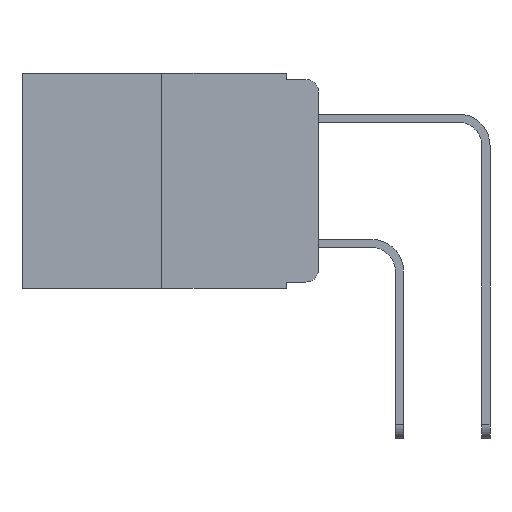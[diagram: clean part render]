
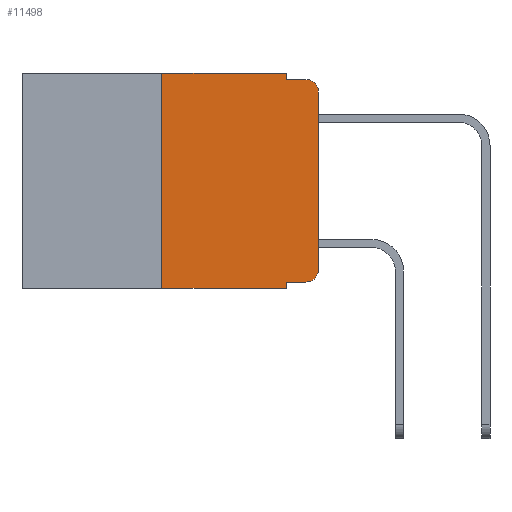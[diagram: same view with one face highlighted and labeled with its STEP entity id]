
A CAD part, left-side view. The second image highlights one B-rep face of the part: STEP entity #11498.
In plain terms, the highlighted planar face has unit normal (-1, 0, 0).
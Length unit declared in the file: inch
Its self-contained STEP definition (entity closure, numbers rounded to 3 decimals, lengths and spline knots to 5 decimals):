
#82 = CARTESIAN_POINT ( 'NONE',  ( 0., 0.051, -0.01 ) ) ;
#469 = CARTESIAN_POINT ( 'NONE',  ( 0., 0.051, -0.333 ) ) ;
#760 = CIRCLE ( 'NONE', #11739, 0.02 ) ;
#832 = PLANE ( 'NONE',  #13525 ) ;
#1111 = EDGE_CURVE ( 'NONE', #13095, #7187, #3518, .T. ) ;
#1128 = ORIENTED_EDGE ( 'NONE', *, *, #9737, .F. ) ;
#1311 = VECTOR ( 'NONE', #10283, 39.37008 ) ;
#1723 = FACE_OUTER_BOUND ( 'NONE', #11784, .T. ) ;
#1800 = EDGE_CURVE ( 'NONE', #10141, #4772, #9819, .T. ) ;
#1827 = CARTESIAN_POINT ( 'NONE',  ( 0., 0.25, 0. ) ) ;
#1835 = VERTEX_POINT ( 'NONE', #9747 ) ;
#1875 = DIRECTION ( 'NONE',  ( 1., 0., 0. ) ) ;
#1890 = DIRECTION ( 'NONE',  ( 0., 0., -1. ) ) ;
#1973 = DIRECTION ( 'NONE',  ( -1., 0., 0. ) ) ;
#2026 = CIRCLE ( 'NONE', #10106, 0.02 ) ;
#2118 = VECTOR ( 'NONE', #4990, 39.37008 ) ;
#2824 = CARTESIAN_POINT ( 'NONE',  ( 0., 0.473, -0.343 ) ) ;
#2964 = DIRECTION ( 'NONE',  ( 0., 0., -1. ) ) ;
#3277 = CARTESIAN_POINT ( 'NONE',  ( 0., 0.02, -0.03 ) ) ;
#3474 = CARTESIAN_POINT ( 'NONE',  ( 0., 0.02, -0.01 ) ) ;
#3518 = LINE ( 'NONE', #2824, #6738 ) ;
#3554 = ORIENTED_EDGE ( 'NONE', *, *, #1800, .F. ) ;
#3802 = CARTESIAN_POINT ( 'NONE',  ( 0., 0.25, 0. ) ) ;
#3855 = EDGE_CURVE ( 'NONE', #10721, #7913, #8476, .T. ) ;
#3869 = ORIENTED_EDGE ( 'NONE', *, *, #1111, .T. ) ;
#4081 = CARTESIAN_POINT ( 'NONE',  ( 0., 0., 0. ) ) ;
#4086 = CARTESIAN_POINT ( 'NONE',  ( 0., 0., -0.03 ) ) ;
#4179 = VECTOR ( 'NONE', #13502, 39.37008 ) ;
#4673 = EDGE_CURVE ( 'NONE', #10721, #7187, #9761, .T. ) ;
#4772 = VERTEX_POINT ( 'NONE', #3474 ) ;
#4841 = CARTESIAN_POINT ( 'NONE',  ( 0., 0.051, -0.01 ) ) ;
#4990 = DIRECTION ( 'NONE',  ( 0., 0., 1. ) ) ;
#5508 = ORIENTED_EDGE ( 'NONE', *, *, #3855, .T. ) ;
#5948 = EDGE_CURVE ( 'NONE', #7913, #6942, #760, .T. ) ;
#5990 = LINE ( 'NONE', #4081, #13233 ) ;
#6186 = EDGE_CURVE ( 'NONE', #12694, #4772, #2026, .T. ) ;
#6331 = VECTOR ( 'NONE', #9337, 39.37008 ) ;
#6393 = EDGE_CURVE ( 'NONE', #12524, #1835, #7195, .T. ) ;
#6719 = ORIENTED_EDGE ( 'NONE', *, *, #6393, .F. ) ;
#6738 = VECTOR ( 'NONE', #10965, 39.37008 ) ;
#6851 = CARTESIAN_POINT ( 'NONE',  ( 0., 0.02, -0.333 ) ) ;
#6942 = VERTEX_POINT ( 'NONE', #10192 ) ;
#7187 = VERTEX_POINT ( 'NONE', #8630 ) ;
#7195 = LINE ( 'NONE', #11316, #12356 ) ;
#7700 = EDGE_CURVE ( 'NONE', #6942, #12694, #5990, .T. ) ;
#7761 = ORIENTED_EDGE ( 'NONE', *, *, #5948, .T. ) ;
#7913 = VERTEX_POINT ( 'NONE', #6851 ) ;
#8254 = CARTESIAN_POINT ( 'NONE',  ( 0., 0.473, 0. ) ) ;
#8351 = CARTESIAN_POINT ( 'NONE',  ( 0., 0.02, -0.313 ) ) ;
#8476 = LINE ( 'NONE', #9762, #6331 ) ;
#8619 = DIRECTION ( 'NONE',  ( 0., 0., -1. ) ) ;
#8630 = CARTESIAN_POINT ( 'NONE',  ( 0., 0.051, -0.343 ) ) ;
#9099 = EDGE_CURVE ( 'NONE', #1835, #10141, #13193, .T. ) ;
#9213 = CARTESIAN_POINT ( 'NONE',  ( 0., 0.051, 0. ) ) ;
#9308 = DIRECTION ( 'NONE',  ( 0., 0., -1. ) ) ;
#9337 = DIRECTION ( 'NONE',  ( 0., -1., 0. ) ) ;
#9737 = EDGE_CURVE ( 'NONE', #13095, #12524, #13197, .T. ) ;
#9747 = CARTESIAN_POINT ( 'NONE',  ( 0., 0.051, 0. ) ) ;
#9761 = LINE ( 'NONE', #9213, #1311 ) ;
#9762 = CARTESIAN_POINT ( 'NONE',  ( 0., 0.051, -0.333 ) ) ;
#9772 = VECTOR ( 'NONE', #1890, 39.37008 ) ;
#9819 = LINE ( 'NONE', #82, #4179 ) ;
#10106 = AXIS2_PLACEMENT_3D ( 'NONE', #3277, #10681, #8619 ) ;
#10141 = VERTEX_POINT ( 'NONE', #4841 ) ;
#10192 = CARTESIAN_POINT ( 'NONE',  ( 0., 0., -0.313 ) ) ;
#10283 = DIRECTION ( 'NONE',  ( 0., 0., -1. ) ) ;
#10459 = DIRECTION ( 'NONE',  ( 0., 0., 1. ) ) ;
#10681 = DIRECTION ( 'NONE',  ( -1., 0., 0. ) ) ;
#10721 = VERTEX_POINT ( 'NONE', #469 ) ;
#10751 = ORIENTED_EDGE ( 'NONE', *, *, #4673, .F. ) ;
#10965 = DIRECTION ( 'NONE',  ( 0., -1., 0. ) ) ;
#11069 = CARTESIAN_POINT ( 'NONE',  ( 0., 0.25, -0.343 ) ) ;
#11316 = CARTESIAN_POINT ( 'NONE',  ( 0., 0.473, 0. ) ) ;
#11397 = ORIENTED_EDGE ( 'NONE', *, *, #9099, .F. ) ;
#11498 = ADVANCED_FACE ( 'NONE', ( #1723 ), #832, .F. ) ;
#11520 = ORIENTED_EDGE ( 'NONE', *, *, #7700, .T. ) ;
#11739 = AXIS2_PLACEMENT_3D ( 'NONE', #8351, #1973, #2964 ) ;
#11784 = EDGE_LOOP ( 'NONE', ( #11520, #12998, #3554, #11397, #6719, #1128, #3869, #10751, #5508, #7761 ) ) ;
#12355 = CARTESIAN_POINT ( 'NONE',  ( 0., 0.051, 0. ) ) ;
#12356 = VECTOR ( 'NONE', #12388, 39.37008 ) ;
#12388 = DIRECTION ( 'NONE',  ( 0., -1., 0. ) ) ;
#12524 = VERTEX_POINT ( 'NONE', #3802 ) ;
#12694 = VERTEX_POINT ( 'NONE', #4086 ) ;
#12998 = ORIENTED_EDGE ( 'NONE', *, *, #6186, .T. ) ;
#13095 = VERTEX_POINT ( 'NONE', #11069 ) ;
#13193 = LINE ( 'NONE', #12355, #9772 ) ;
#13197 = LINE ( 'NONE', #1827, #2118 ) ;
#13233 = VECTOR ( 'NONE', #10459, 39.37008 ) ;
#13502 = DIRECTION ( 'NONE',  ( 0., -1., 0. ) ) ;
#13525 = AXIS2_PLACEMENT_3D ( 'NONE', #8254, #1875, #9308 ) ;
